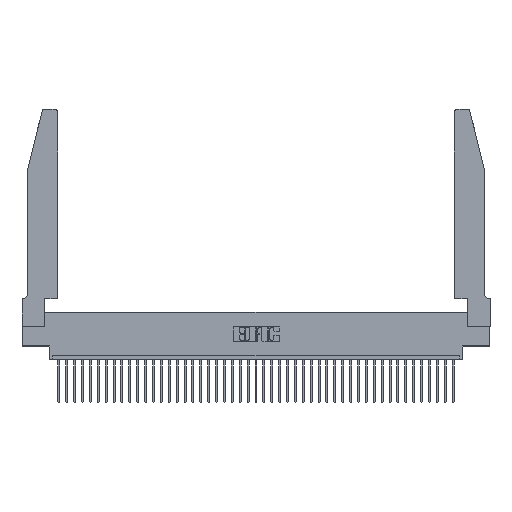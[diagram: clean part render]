
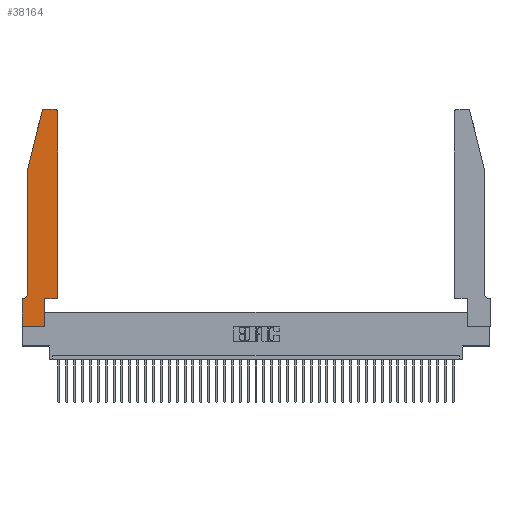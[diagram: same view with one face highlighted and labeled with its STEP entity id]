
A CAD part, top view. The second image highlights one B-rep face of the part: STEP entity #38164.
In plain terms, the highlighted planar face has unit normal (0, 0, 1).
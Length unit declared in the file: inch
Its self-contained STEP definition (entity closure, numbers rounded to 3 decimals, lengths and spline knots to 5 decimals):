
#76 = VECTOR ( 'NONE', #22423, 39.37008 ) ;
#127 = VERTEX_POINT ( 'NONE', #17166 ) ;
#207 = DIRECTION ( 'NONE',  ( 0., 0., 1. ) ) ;
#214 = EDGE_CURVE ( 'NONE', #19631, #38059, #22694, .T. ) ;
#808 = DIRECTION ( 'NONE',  ( -0.239, -0.971, 0. ) ) ;
#1128 = LINE ( 'NONE', #12866, #76 ) ;
#1461 = LINE ( 'NONE', #3855, #9557 ) ;
#1984 = VERTEX_POINT ( 'NONE', #11035 ) ;
#2005 = CIRCLE ( 'NONE', #34305, 0.03 ) ;
#2195 = AXIS2_PLACEMENT_3D ( 'NONE', #29734, #207, #23208 ) ;
#2260 = EDGE_CURVE ( 'NONE', #10093, #14298, #20766, .T. ) ;
#2595 = EDGE_CURVE ( 'NONE', #127, #14427, #10521, .T. ) ;
#2884 = EDGE_CURVE ( 'NONE', #28516, #10093, #26787, .T. ) ;
#3007 = EDGE_CURVE ( 'NONE', #21661, #36639, #24283, .T. ) ;
#3769 = EDGE_CURVE ( 'NONE', #14298, #23088, #16568, .T. ) ;
#3855 = CARTESIAN_POINT ( 'NONE',  ( 0.2605, 2.75, 0.37 ) ) ;
#4101 = EDGE_LOOP ( 'NONE', ( #10421, #20359, #36858, #24904, #4570, #38960, #9644, #4476, #14200, #22270, #41529, #5104 ) ) ;
#4119 = EDGE_CURVE ( 'NONE', #1984, #28516, #33220, .T. ) ;
#4182 = CARTESIAN_POINT ( 'NONE',  ( 0.2865, 0.35, 0.37 ) ) ;
#4391 = VECTOR ( 'NONE', #808, 39.37008 ) ;
#4476 = ORIENTED_EDGE ( 'NONE', *, *, #3769, .T. ) ;
#4570 = ORIENTED_EDGE ( 'NONE', *, *, #4119, .T. ) ;
#5104 = ORIENTED_EDGE ( 'NONE', *, *, #2595, .T. ) ;
#6604 = CARTESIAN_POINT ( 'NONE',  ( 0.0055, 0.42, 0.37 ) ) ;
#6836 = DIRECTION ( 'NONE',  ( 0., 1., 0. ) ) ;
#7237 = DIRECTION ( 'NONE',  ( -1., 0., 0. ) ) ;
#7895 = VECTOR ( 'NONE', #12255, 39.37008 ) ;
#8342 = CARTESIAN_POINT ( 'NONE',  ( 0.4505, 0.35, 0.37 ) ) ;
#8649 = VECTOR ( 'NONE', #34445, 39.37008 ) ;
#9009 = DIRECTION ( 'NONE',  ( 0., 0., 1. ) ) ;
#9557 = VECTOR ( 'NONE', #7237, 39.37008 ) ;
#9644 = ORIENTED_EDGE ( 'NONE', *, *, #2260, .T. ) ;
#10093 = VERTEX_POINT ( 'NONE', #19698 ) ;
#10421 = ORIENTED_EDGE ( 'NONE', *, *, #33425, .T. ) ;
#10521 = CIRCLE ( 'NONE', #31916, 0.03 ) ;
#10559 = CARTESIAN_POINT ( 'NONE',  ( 0.4505, 0.35, 0.37 ) ) ;
#11035 = CARTESIAN_POINT ( 'NONE',  ( 0.0755, 0.42, 0.37 ) ) ;
#11195 = EDGE_CURVE ( 'NONE', #23088, #21661, #22343, .T. ) ;
#11251 = CARTESIAN_POINT ( 'NONE',  ( 0.4205, 2.72, 0.37 ) ) ;
#12255 = DIRECTION ( 'NONE',  ( 1., 0., 0. ) ) ;
#12866 = CARTESIAN_POINT ( 'NONE',  ( 0.0755, 2., 0.37 ) ) ;
#13559 = CARTESIAN_POINT ( 'NONE',  ( 0., 0., 0.37 ) ) ;
#14200 = ORIENTED_EDGE ( 'NONE', *, *, #11195, .T. ) ;
#14298 = VERTEX_POINT ( 'NONE', #30052 ) ;
#14427 = VERTEX_POINT ( 'NONE', #35971 ) ;
#14594 = VECTOR ( 'NONE', #16336, 39.37008 ) ;
#15577 = EDGE_CURVE ( 'NONE', #38059, #1984, #1128, .T. ) ;
#15715 = VECTOR ( 'NONE', #6836, 39.37008 ) ;
#16336 = DIRECTION ( 'NONE',  ( -1., 0., 0. ) ) ;
#16410 = CARTESIAN_POINT ( 'NONE',  ( 0.2865, 0.35, 0.37 ) ) ;
#16568 = LINE ( 'NONE', #25377, #7895 ) ;
#17166 = CARTESIAN_POINT ( 'NONE',  ( 0.4505, 2.72, 0.37 ) ) ;
#17325 = AXIS2_PLACEMENT_3D ( 'NONE', #6604, #39114, #19695 ) ;
#18688 = VECTOR ( 'NONE', #30773, 39.37008 ) ;
#19631 = VERTEX_POINT ( 'NONE', #36415 ) ;
#19695 = DIRECTION ( 'NONE',  ( -1., 0., 0. ) ) ;
#19698 = CARTESIAN_POINT ( 'NONE',  ( 0., 0.35, 0.37 ) ) ;
#20359 = ORIENTED_EDGE ( 'NONE', *, *, #39303, .T. ) ;
#20752 = CARTESIAN_POINT ( 'NONE',  ( 0.0755, 2., 0.37 ) ) ;
#20766 = LINE ( 'NONE', #13559, #33403 ) ;
#21661 = VERTEX_POINT ( 'NONE', #4182 ) ;
#22270 = ORIENTED_EDGE ( 'NONE', *, *, #3007, .T. ) ;
#22316 = CARTESIAN_POINT ( 'NONE',  ( 0.0755, 0.35, 0.37 ) ) ;
#22343 = LINE ( 'NONE', #16410, #15715 ) ;
#22423 = DIRECTION ( 'NONE',  ( 0., -1., 0. ) ) ;
#22694 = LINE ( 'NONE', #33701, #4391 ) ;
#23088 = VERTEX_POINT ( 'NONE', #40954 ) ;
#23208 = DIRECTION ( 'NONE',  ( 1., 0., 0. ) ) ;
#24283 = LINE ( 'NONE', #31187, #18688 ) ;
#24904 = ORIENTED_EDGE ( 'NONE', *, *, #15577, .T. ) ;
#25377 = CARTESIAN_POINT ( 'NONE',  ( 0., 0., 0.37 ) ) ;
#26787 = LINE ( 'NONE', #22316, #14594 ) ;
#28516 = VERTEX_POINT ( 'NONE', #35954 ) ;
#29734 = CARTESIAN_POINT ( 'NONE',  ( 0., 0.35, 0.37 ) ) ;
#30052 = CARTESIAN_POINT ( 'NONE',  ( 0., 0., 0.37 ) ) ;
#30773 = DIRECTION ( 'NONE',  ( 1., 0., 0. ) ) ;
#31187 = CARTESIAN_POINT ( 'NONE',  ( 0.4505, 0.35, 0.37 ) ) ;
#31916 = AXIS2_PLACEMENT_3D ( 'NONE', #11251, #40063, #33935 ) ;
#32215 = VERTEX_POINT ( 'NONE', #40491 ) ;
#33220 = CIRCLE ( 'NONE', #17325, 0.07 ) ;
#33403 = VECTOR ( 'NONE', #40095, 39.37008 ) ;
#33425 = EDGE_CURVE ( 'NONE', #14427, #32215, #1461, .T. ) ;
#33701 = CARTESIAN_POINT ( 'NONE',  ( 0.0755, 2., 0.37 ) ) ;
#33935 = DIRECTION ( 'NONE',  ( 1., 0., 0. ) ) ;
#34305 = AXIS2_PLACEMENT_3D ( 'NONE', #41840, #9009, #41973 ) ;
#34445 = DIRECTION ( 'NONE',  ( 0., 1., 0. ) ) ;
#35954 = CARTESIAN_POINT ( 'NONE',  ( 0.0055, 0.35, 0.37 ) ) ;
#35971 = CARTESIAN_POINT ( 'NONE',  ( 0.4205, 2.75, 0.37 ) ) ;
#36415 = CARTESIAN_POINT ( 'NONE',  ( 0.25487, 2.72718, 0.37 ) ) ;
#36587 = LINE ( 'NONE', #8342, #8649 ) ;
#36639 = VERTEX_POINT ( 'NONE', #10559 ) ;
#36858 = ORIENTED_EDGE ( 'NONE', *, *, #214, .T. ) ;
#38059 = VERTEX_POINT ( 'NONE', #20752 ) ;
#38063 = EDGE_CURVE ( 'NONE', #36639, #127, #36587, .T. ) ;
#38164 = ADVANCED_FACE ( 'NONE', ( #39661 ), #38787, .T. ) ;
#38787 = PLANE ( 'NONE',  #2195 ) ;
#38960 = ORIENTED_EDGE ( 'NONE', *, *, #2884, .T. ) ;
#39114 = DIRECTION ( 'NONE',  ( 0., 0., -1. ) ) ;
#39303 = EDGE_CURVE ( 'NONE', #32215, #19631, #2005, .T. ) ;
#39661 = FACE_OUTER_BOUND ( 'NONE', #4101, .T. ) ;
#40063 = DIRECTION ( 'NONE',  ( 0., 0., 1. ) ) ;
#40095 = DIRECTION ( 'NONE',  ( 0., -1., 0. ) ) ;
#40491 = CARTESIAN_POINT ( 'NONE',  ( 0.284, 2.75, 0.37 ) ) ;
#40954 = CARTESIAN_POINT ( 'NONE',  ( 0.2865, 0., 0.37 ) ) ;
#41529 = ORIENTED_EDGE ( 'NONE', *, *, #38063, .T. ) ;
#41840 = CARTESIAN_POINT ( 'NONE',  ( 0.284, 2.72, 0.37 ) ) ;
#41973 = DIRECTION ( 'NONE',  ( 1., 0., 0. ) ) ;
